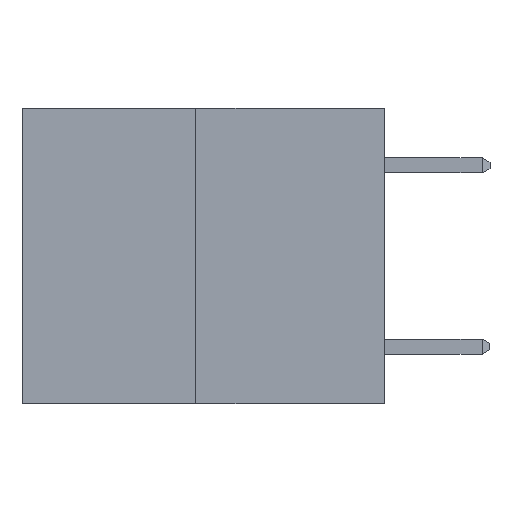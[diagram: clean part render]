
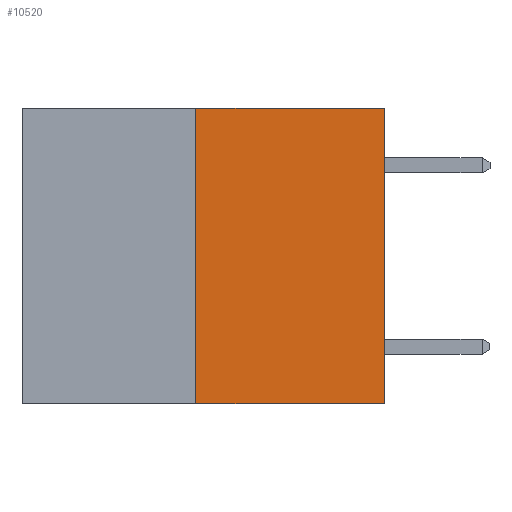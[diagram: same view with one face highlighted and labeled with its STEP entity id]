
A CAD part, left-side view. The second image highlights one B-rep face of the part: STEP entity #10520.
In plain terms, the highlighted planar face has unit normal (-1, 0, 0).
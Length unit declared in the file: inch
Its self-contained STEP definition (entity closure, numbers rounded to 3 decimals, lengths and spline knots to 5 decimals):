
#23 = DIRECTION ( 'NONE',  ( 0., 0., 1. ) ) ;
#913 = LINE ( 'NONE', #9798, #1954 ) ;
#1954 = VECTOR ( 'NONE', #23, 39.37008 ) ;
#2018 = CARTESIAN_POINT ( 'NONE',  ( 0., 0.312, 0. ) ) ;
#2492 = VERTEX_POINT ( 'NONE', #2018 ) ;
#2505 = DIRECTION ( 'NONE',  ( 0., -1., 0. ) ) ;
#2548 = EDGE_CURVE ( 'NONE', #9770, #2492, #913, .T. ) ;
#2570 = VERTEX_POINT ( 'NONE', #6672 ) ;
#2585 = CARTESIAN_POINT ( 'NONE',  ( 0., 0., 0. ) ) ;
#2817 = EDGE_CURVE ( 'NONE', #9770, #2570, #9897, .T. ) ;
#3133 = ORIENTED_EDGE ( 'NONE', *, *, #4470, .T. ) ;
#3676 = DIRECTION ( 'NONE',  ( 0., 0., 1. ) ) ;
#4470 = EDGE_CURVE ( 'NONE', #2570, #5987, #11230, .T. ) ;
#4879 = FACE_OUTER_BOUND ( 'NONE', #13120, .T. ) ;
#4938 = CARTESIAN_POINT ( 'NONE',  ( 0., 0.6, 0. ) ) ;
#5396 = CARTESIAN_POINT ( 'NONE',  ( 0., 0.312, -0.49 ) ) ;
#5987 = VERTEX_POINT ( 'NONE', #2585 ) ;
#6047 = DIRECTION ( 'NONE',  ( 0., 0., -1. ) ) ;
#6387 = VECTOR ( 'NONE', #6979, 39.37008 ) ;
#6672 = CARTESIAN_POINT ( 'NONE',  ( 0., 0., -0.49 ) ) ;
#6799 = ORIENTED_EDGE ( 'NONE', *, *, #12104, .F. ) ;
#6979 = DIRECTION ( 'NONE',  ( 0., -1., 0. ) ) ;
#7022 = AXIS2_PLACEMENT_3D ( 'NONE', #4938, #12735, #6047 ) ;
#8640 = VECTOR ( 'NONE', #3676, 39.37008 ) ;
#8967 = ORIENTED_EDGE ( 'NONE', *, *, #2817, .T. ) ;
#9770 = VERTEX_POINT ( 'NONE', #5396 ) ;
#9798 = CARTESIAN_POINT ( 'NONE',  ( 0., 0.312, -0.49 ) ) ;
#9897 = LINE ( 'NONE', #11464, #13735 ) ;
#10070 = LINE ( 'NONE', #11410, #6387 ) ;
#10520 = ADVANCED_FACE ( 'NONE', ( #4879 ), #11606, .F. ) ;
#11230 = LINE ( 'NONE', #12491, #8640 ) ;
#11410 = CARTESIAN_POINT ( 'NONE',  ( 0., 0.6, 0. ) ) ;
#11464 = CARTESIAN_POINT ( 'NONE',  ( 0., 0.6, -0.49 ) ) ;
#11606 = PLANE ( 'NONE',  #7022 ) ;
#12104 = EDGE_CURVE ( 'NONE', #2492, #5987, #10070, .T. ) ;
#12491 = CARTESIAN_POINT ( 'NONE',  ( 0., 0., 0. ) ) ;
#12735 = DIRECTION ( 'NONE',  ( 1., 0., 0. ) ) ;
#13107 = ORIENTED_EDGE ( 'NONE', *, *, #2548, .F. ) ;
#13120 = EDGE_LOOP ( 'NONE', ( #13107, #8967, #3133, #6799 ) ) ;
#13735 = VECTOR ( 'NONE', #2505, 39.37008 ) ;
